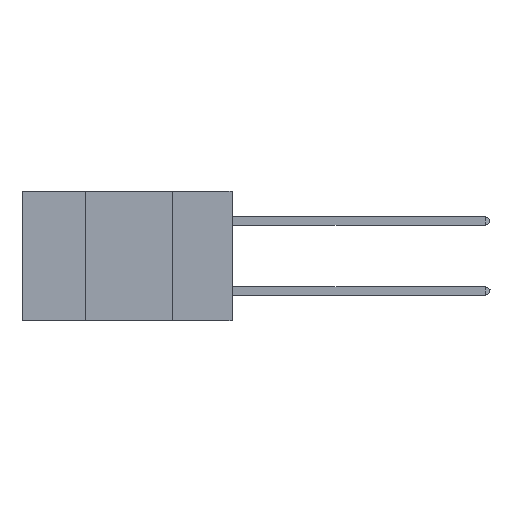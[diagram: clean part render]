
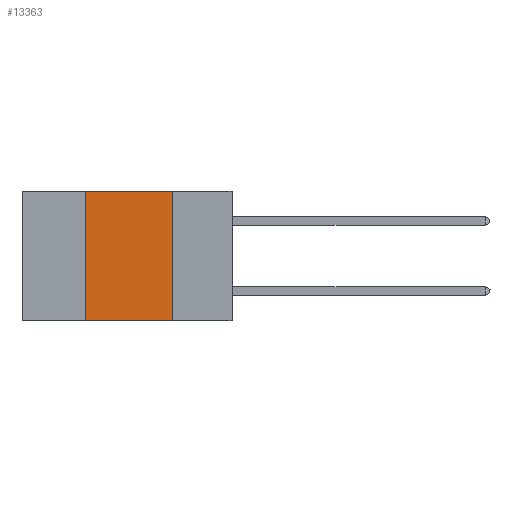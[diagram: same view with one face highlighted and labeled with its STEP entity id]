
A CAD part, left-side view. The second image highlights one B-rep face of the part: STEP entity #13363.
In plain terms, the highlighted planar face has unit normal (-1, 0, 0).
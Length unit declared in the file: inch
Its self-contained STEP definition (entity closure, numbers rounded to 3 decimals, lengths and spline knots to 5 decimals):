
#479 = LINE ( 'NONE', #1729, #13864 ) ;
#483 = DIRECTION ( 'NONE',  ( 0., 0., -1. ) ) ;
#563 = PLANE ( 'NONE',  #12438 ) ;
#624 = EDGE_LOOP ( 'NONE', ( #11215, #8594, #18084, #19519 ) ) ;
#1232 = DIRECTION ( 'NONE',  ( 0., 0., -1. ) ) ;
#1729 = CARTESIAN_POINT ( 'NONE',  ( 0., 0.42, 0. ) ) ;
#1748 = VERTEX_POINT ( 'NONE', #19026 ) ;
#1882 = VERTEX_POINT ( 'NONE', #5794 ) ;
#3162 = VECTOR ( 'NONE', #10267, 39.37008 ) ;
#3279 = CARTESIAN_POINT ( 'NONE',  ( 0., 0.42, 0. ) ) ;
#4358 = CARTESIAN_POINT ( 'NONE',  ( 0., 0.17, 0. ) ) ;
#5327 = DIRECTION ( 'NONE',  ( 0., -1., 0. ) ) ;
#5794 = CARTESIAN_POINT ( 'NONE',  ( 0., 0.42, -0.37 ) ) ;
#6574 = FACE_OUTER_BOUND ( 'NONE', #624, .T. ) ;
#6847 = LINE ( 'NONE', #9804, #14472 ) ;
#7021 = EDGE_CURVE ( 'NONE', #1882, #18543, #479, .T. ) ;
#7734 = EDGE_CURVE ( 'NONE', #18543, #1748, #6847, .T. ) ;
#8256 = VECTOR ( 'NONE', #1232, 39.37008 ) ;
#8594 = ORIENTED_EDGE ( 'NONE', *, *, #7734, .F. ) ;
#9662 = DIRECTION ( 'NONE',  ( 1., 0., 0. ) ) ;
#9804 = CARTESIAN_POINT ( 'NONE',  ( 0., 0.6, 0. ) ) ;
#10267 = DIRECTION ( 'NONE',  ( 0., -1., 0. ) ) ;
#10931 = DIRECTION ( 'NONE',  ( 0., 0., 1. ) ) ;
#11215 = ORIENTED_EDGE ( 'NONE', *, *, #18284, .F. ) ;
#11593 = CARTESIAN_POINT ( 'NONE',  ( 0., 0.6, -0.37 ) ) ;
#11597 = LINE ( 'NONE', #4358, #8256 ) ;
#12225 = VERTEX_POINT ( 'NONE', #17277 ) ;
#12438 = AXIS2_PLACEMENT_3D ( 'NONE', #14113, #9662, #483 ) ;
#13363 = ADVANCED_FACE ( 'NONE', ( #6574 ), #563, .F. ) ;
#13864 = VECTOR ( 'NONE', #10931, 39.37008 ) ;
#13914 = LINE ( 'NONE', #11593, #3162 ) ;
#14113 = CARTESIAN_POINT ( 'NONE',  ( 0., 0.6, 0. ) ) ;
#14472 = VECTOR ( 'NONE', #5327, 39.37008 ) ;
#17277 = CARTESIAN_POINT ( 'NONE',  ( 0., 0.17, -0.37 ) ) ;
#18084 = ORIENTED_EDGE ( 'NONE', *, *, #7021, .F. ) ;
#18284 = EDGE_CURVE ( 'NONE', #1748, #12225, #11597, .T. ) ;
#18543 = VERTEX_POINT ( 'NONE', #3279 ) ;
#19026 = CARTESIAN_POINT ( 'NONE',  ( 0., 0.17, 0. ) ) ;
#19519 = ORIENTED_EDGE ( 'NONE', *, *, #19658, .T. ) ;
#19658 = EDGE_CURVE ( 'NONE', #1882, #12225, #13914, .T. ) ;
